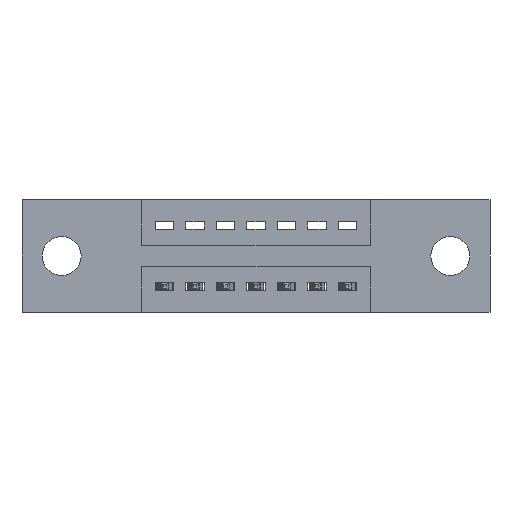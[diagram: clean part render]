
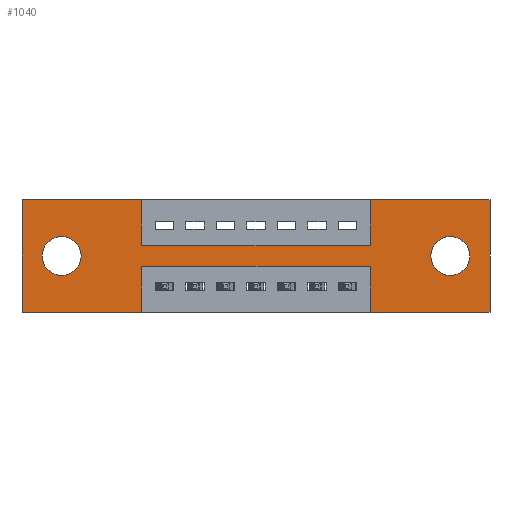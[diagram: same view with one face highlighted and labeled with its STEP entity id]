
A CAD part, front view. The second image highlights one B-rep face of the part: STEP entity #1040.
In plain terms, the highlighted planar face has unit normal (0, -1, 0).
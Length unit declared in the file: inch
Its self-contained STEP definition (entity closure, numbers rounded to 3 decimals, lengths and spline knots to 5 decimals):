
#13 = ORIENTED_EDGE ( 'NONE', *, *, #930, .F. ) ;
#37 = EDGE_LOOP ( 'NONE', ( #1287, #4074 ) ) ;
#64 = ORIENTED_EDGE ( 'NONE', *, *, #7408, .F. ) ;
#98 = EDGE_CURVE ( 'NONE', #4302, #9418, #4184, .T. ) ;
#150 = ORIENTED_EDGE ( 'NONE', *, *, #4698, .F. ) ;
#227 = EDGE_CURVE ( 'NONE', #2777, #2372, #1159, .T. ) ;
#406 = CARTESIAN_POINT ( 'NONE',  ( 0., 0., -0.37 ) ) ;
#427 = VERTEX_POINT ( 'NONE', #1248 ) ;
#436 = CARTESIAN_POINT ( 'NONE',  ( 1.535, 0., 0. ) ) ;
#468 = CARTESIAN_POINT ( 'NONE',  ( 0.13, 0., -0.185 ) ) ;
#496 = VECTOR ( 'NONE', #4146, 39.37008 ) ;
#608 = LINE ( 'NONE', #4464, #6277 ) ;
#708 = LINE ( 'NONE', #4298, #6511 ) ;
#757 = EDGE_LOOP ( 'NONE', ( #2633, #3008, #64, #13, #8684, #150, #6208, #8239, #4234, #3130, #5992, #6632 ) ) ;
#899 = CARTESIAN_POINT ( 'NONE',  ( 0., 0., 0. ) ) ;
#921 = VECTOR ( 'NONE', #1873, 39.37008 ) ;
#930 = EDGE_CURVE ( 'NONE', #2372, #427, #7424, .T. ) ;
#961 = CARTESIAN_POINT ( 'NONE',  ( 1.1425, 0., -0.37 ) ) ;
#1004 = AXIS2_PLACEMENT_3D ( 'NONE', #7218, #6342, #4153 ) ;
#1040 = ADVANCED_FACE ( 'NONE', ( #2474, #8392, #2835 ), #1834, .T. ) ;
#1041 = CARTESIAN_POINT ( 'NONE',  ( 0., 0., 0. ) ) ;
#1159 = LINE ( 'NONE', #436, #921 ) ;
#1248 = CARTESIAN_POINT ( 'NONE',  ( 1.1425, 0., -0.37 ) ) ;
#1250 = LINE ( 'NONE', #1748, #2327 ) ;
#1287 = ORIENTED_EDGE ( 'NONE', *, *, #7124, .T. ) ;
#1358 = CARTESIAN_POINT ( 'NONE',  ( 0.3925, 0., -0.22 ) ) ;
#1368 = AXIS2_PLACEMENT_3D ( 'NONE', #468, #6627, #7097 ) ;
#1439 = LINE ( 'NONE', #1041, #3255 ) ;
#1708 = EDGE_CURVE ( 'NONE', #8791, #3471, #3547, .T. ) ;
#1748 = CARTESIAN_POINT ( 'NONE',  ( 0., 0., -0.37 ) ) ;
#1794 = VECTOR ( 'NONE', #4101, 39.37008 ) ;
#1834 = PLANE ( 'NONE',  #1004 ) ;
#1863 = EDGE_CURVE ( 'NONE', #8127, #2615, #1250, .T. ) ;
#1873 = DIRECTION ( 'NONE',  ( 0., 0., -1. ) ) ;
#1992 = DIRECTION ( 'NONE',  ( 0., 0., -1. ) ) ;
#2071 = LINE ( 'NONE', #961, #2185 ) ;
#2158 = CARTESIAN_POINT ( 'NONE',  ( 0.13, 0., -0.185 ) ) ;
#2185 = VECTOR ( 'NONE', #3979, 39.37008 ) ;
#2227 = EDGE_CURVE ( 'NONE', #9117, #6473, #5711, .T. ) ;
#2327 = VECTOR ( 'NONE', #4006, 39.37008 ) ;
#2372 = VERTEX_POINT ( 'NONE', #3889 ) ;
#2406 = ORIENTED_EDGE ( 'NONE', *, *, #8415, .T. ) ;
#2448 = LINE ( 'NONE', #5580, #6307 ) ;
#2474 = FACE_BOUND ( 'NONE', #37, .T. ) ;
#2488 = EDGE_CURVE ( 'NONE', #5044, #3603, #2448, .T. ) ;
#2532 = CARTESIAN_POINT ( 'NONE',  ( 0.3925, 0., -0.37 ) ) ;
#2615 = VERTEX_POINT ( 'NONE', #406 ) ;
#2619 = CARTESIAN_POINT ( 'NONE',  ( 1.1425, 0., -0.22 ) ) ;
#2633 = ORIENTED_EDGE ( 'NONE', *, *, #5518, .F. ) ;
#2777 = VERTEX_POINT ( 'NONE', #6695 ) ;
#2835 = FACE_OUTER_BOUND ( 'NONE', #757, .T. ) ;
#2851 = CARTESIAN_POINT ( 'NONE',  ( 0., 0., 0. ) ) ;
#2862 = LINE ( 'NONE', #2532, #1794 ) ;
#2932 = VECTOR ( 'NONE', #8923, 39.37008 ) ;
#2945 = CARTESIAN_POINT ( 'NONE',  ( 1.405, 0., -0.185 ) ) ;
#3008 = ORIENTED_EDGE ( 'NONE', *, *, #1708, .F. ) ;
#3130 = ORIENTED_EDGE ( 'NONE', *, *, #7451, .F. ) ;
#3255 = VECTOR ( 'NONE', #9920, 39.37008 ) ;
#3471 = VERTEX_POINT ( 'NONE', #1358 ) ;
#3547 = LINE ( 'NONE', #4265, #2932 ) ;
#3603 = VERTEX_POINT ( 'NONE', #8441 ) ;
#3668 = DIRECTION ( 'NONE',  ( 1., 0., 0. ) ) ;
#3889 = CARTESIAN_POINT ( 'NONE',  ( 1.535, 0., -0.37 ) ) ;
#3895 = VECTOR ( 'NONE', #9505, 39.37008 ) ;
#3908 = EDGE_CURVE ( 'NONE', #3603, #4909, #8341, .T. ) ;
#3979 = DIRECTION ( 'NONE',  ( 0., 0., 1. ) ) ;
#4006 = DIRECTION ( 'NONE',  ( -1., 0., 0. ) ) ;
#4074 = ORIENTED_EDGE ( 'NONE', *, *, #98, .T. ) ;
#4101 = DIRECTION ( 'NONE',  ( 0., 0., -1. ) ) ;
#4146 = DIRECTION ( 'NONE',  ( 0., 0., 1. ) ) ;
#4153 = DIRECTION ( 'NONE',  ( 0., 0., -1. ) ) ;
#4184 = CIRCLE ( 'NONE', #4694, 0.064 ) ;
#4187 = CARTESIAN_POINT ( 'NONE',  ( 0.3925, 0., -0.15 ) ) ;
#4234 = ORIENTED_EDGE ( 'NONE', *, *, #9354, .F. ) ;
#4265 = CARTESIAN_POINT ( 'NONE',  ( 0.3925, 0., -0.22 ) ) ;
#4298 = CARTESIAN_POINT ( 'NONE',  ( 0.3925, 0., 0. ) ) ;
#4302 = VERTEX_POINT ( 'NONE', #5302 ) ;
#4333 = CARTESIAN_POINT ( 'NONE',  ( 1.405, 0., -0.121 ) ) ;
#4447 = ORIENTED_EDGE ( 'NONE', *, *, #2227, .T. ) ;
#4464 = CARTESIAN_POINT ( 'NONE',  ( 0., 0., 0. ) ) ;
#4670 = CARTESIAN_POINT ( 'NONE',  ( 0., 0., -0.37 ) ) ;
#4679 = VERTEX_POINT ( 'NONE', #2851 ) ;
#4694 = AXIS2_PLACEMENT_3D ( 'NONE', #6440, #4878, #5547 ) ;
#4698 = EDGE_CURVE ( 'NONE', #4909, #2777, #608, .T. ) ;
#4751 = CARTESIAN_POINT ( 'NONE',  ( 1.1425, 0., 0. ) ) ;
#4878 = DIRECTION ( 'NONE',  ( 0., 1., 0. ) ) ;
#4909 = VERTEX_POINT ( 'NONE', #4751 ) ;
#5044 = VERTEX_POINT ( 'NONE', #4187 ) ;
#5302 = CARTESIAN_POINT ( 'NONE',  ( 1.405, 0., -0.249 ) ) ;
#5317 = DIRECTION ( 'NONE',  ( 0., 0., -1. ) ) ;
#5518 = EDGE_CURVE ( 'NONE', #3471, #8127, #2862, .T. ) ;
#5547 = DIRECTION ( 'NONE',  ( 0., 0., -1. ) ) ;
#5580 = CARTESIAN_POINT ( 'NONE',  ( 0.3925, 0., -0.15 ) ) ;
#5711 = CIRCLE ( 'NONE', #9757, 0.064 ) ;
#5951 = DIRECTION ( 'NONE',  ( 0., 1., 0. ) ) ;
#5992 = ORIENTED_EDGE ( 'NONE', *, *, #6107, .F. ) ;
#6107 = EDGE_CURVE ( 'NONE', #2615, #4679, #1439, .T. ) ;
#6208 = ORIENTED_EDGE ( 'NONE', *, *, #3908, .F. ) ;
#6277 = VECTOR ( 'NONE', #3668, 39.37008 ) ;
#6280 = DIRECTION ( 'NONE',  ( 1., 0., 0. ) ) ;
#6307 = VECTOR ( 'NONE', #6280, 39.37008 ) ;
#6342 = DIRECTION ( 'NONE',  ( 0., -1., 0. ) ) ;
#6433 = CARTESIAN_POINT ( 'NONE',  ( 1.1425, 0., 0. ) ) ;
#6440 = CARTESIAN_POINT ( 'NONE',  ( 1.405, 0., -0.185 ) ) ;
#6468 = EDGE_LOOP ( 'NONE', ( #4447, #2406 ) ) ;
#6473 = VERTEX_POINT ( 'NONE', #7988 ) ;
#6511 = VECTOR ( 'NONE', #1992, 39.37008 ) ;
#6627 = DIRECTION ( 'NONE',  ( 0., 1., 0. ) ) ;
#6632 = ORIENTED_EDGE ( 'NONE', *, *, #1863, .F. ) ;
#6654 = LINE ( 'NONE', #899, #3895 ) ;
#6695 = CARTESIAN_POINT ( 'NONE',  ( 1.535, 0., 0. ) ) ;
#6986 = CARTESIAN_POINT ( 'NONE',  ( 0.3925, 0., -0.37 ) ) ;
#7097 = DIRECTION ( 'NONE',  ( 0., 0., 1. ) ) ;
#7124 = EDGE_CURVE ( 'NONE', #9418, #4302, #9605, .T. ) ;
#7125 = CIRCLE ( 'NONE', #1368, 0.064 ) ;
#7218 = CARTESIAN_POINT ( 'NONE',  ( 0., 0., -0.37 ) ) ;
#7408 = EDGE_CURVE ( 'NONE', #427, #8791, #2071, .T. ) ;
#7424 = LINE ( 'NONE', #4670, #9744 ) ;
#7451 = EDGE_CURVE ( 'NONE', #4679, #10017, #6654, .T. ) ;
#7799 = DIRECTION ( 'NONE',  ( -1., 0., 0. ) ) ;
#7916 = CARTESIAN_POINT ( 'NONE',  ( 0.13, 0., -0.121 ) ) ;
#7988 = CARTESIAN_POINT ( 'NONE',  ( 0.13, 0., -0.249 ) ) ;
#8127 = VERTEX_POINT ( 'NONE', #6986 ) ;
#8239 = ORIENTED_EDGE ( 'NONE', *, *, #2488, .F. ) ;
#8341 = LINE ( 'NONE', #6433, #496 ) ;
#8392 = FACE_BOUND ( 'NONE', #6468, .T. ) ;
#8415 = EDGE_CURVE ( 'NONE', #6473, #9117, #7125, .T. ) ;
#8441 = CARTESIAN_POINT ( 'NONE',  ( 1.1425, 0., -0.15 ) ) ;
#8684 = ORIENTED_EDGE ( 'NONE', *, *, #227, .F. ) ;
#8791 = VERTEX_POINT ( 'NONE', #2619 ) ;
#8870 = AXIS2_PLACEMENT_3D ( 'NONE', #2945, #9955, #5317 ) ;
#8923 = DIRECTION ( 'NONE',  ( -1., 0., 0. ) ) ;
#9117 = VERTEX_POINT ( 'NONE', #7916 ) ;
#9143 = DIRECTION ( 'NONE',  ( 0., 0., 1. ) ) ;
#9354 = EDGE_CURVE ( 'NONE', #10017, #5044, #708, .T. ) ;
#9418 = VERTEX_POINT ( 'NONE', #4333 ) ;
#9505 = DIRECTION ( 'NONE',  ( 1., 0., 0. ) ) ;
#9572 = CARTESIAN_POINT ( 'NONE',  ( 0.3925, 0., 0. ) ) ;
#9605 = CIRCLE ( 'NONE', #8870, 0.064 ) ;
#9744 = VECTOR ( 'NONE', #7799, 39.37008 ) ;
#9757 = AXIS2_PLACEMENT_3D ( 'NONE', #2158, #5951, #9143 ) ;
#9920 = DIRECTION ( 'NONE',  ( 0., 0., 1. ) ) ;
#9955 = DIRECTION ( 'NONE',  ( 0., 1., 0. ) ) ;
#10017 = VERTEX_POINT ( 'NONE', #9572 ) ;
